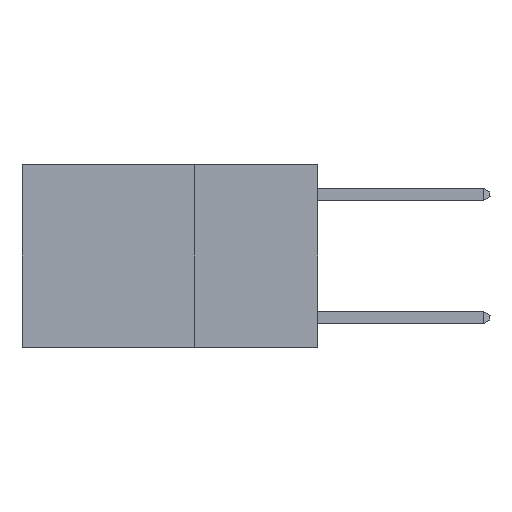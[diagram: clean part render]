
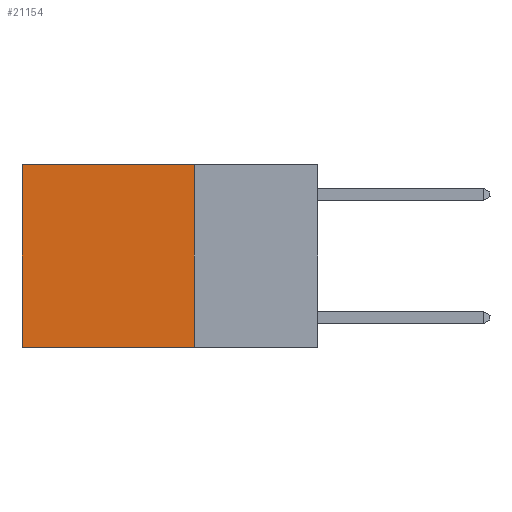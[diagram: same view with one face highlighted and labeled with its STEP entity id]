
A CAD part, left-side view. The second image highlights one B-rep face of the part: STEP entity #21154.
In plain terms, the highlighted planar face has unit normal (-1, 0, 0).
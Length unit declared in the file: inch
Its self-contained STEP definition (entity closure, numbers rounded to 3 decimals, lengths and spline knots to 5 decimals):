
#1165 = VECTOR ( 'NONE', #25791, 39.37008 ) ;
#1932 = VERTEX_POINT ( 'NONE', #30349 ) ;
#2267 = DIRECTION ( 'NONE',  ( 1., 0., 0. ) ) ;
#3977 = LINE ( 'NONE', #15741, #16238 ) ;
#4914 = LINE ( 'NONE', #23691, #30261 ) ;
#5158 = CARTESIAN_POINT ( 'NONE',  ( 0.2625, 0.6, -0.37 ) ) ;
#5174 = VERTEX_POINT ( 'NONE', #22373 ) ;
#7076 = ORIENTED_EDGE ( 'NONE', *, *, #25683, .F. ) ;
#7470 = ORIENTED_EDGE ( 'NONE', *, *, #29866, .T. ) ;
#8504 = VERTEX_POINT ( 'NONE', #5158 ) ;
#8608 = EDGE_CURVE ( 'NONE', #1932, #28725, #10724, .T. ) ;
#9175 = AXIS2_PLACEMENT_3D ( 'NONE', #31660, #2267, #19341 ) ;
#9919 = CARTESIAN_POINT ( 'NONE',  ( 0.2625, 0.6, 0. ) ) ;
#10724 = LINE ( 'NONE', #12882, #29503 ) ;
#12882 = CARTESIAN_POINT ( 'NONE',  ( 0.2625, 0.25, 0. ) ) ;
#14474 = PLANE ( 'NONE',  #9175 ) ;
#15741 = CARTESIAN_POINT ( 'NONE',  ( 0.2625, 0.25, -0.37 ) ) ;
#16238 = VECTOR ( 'NONE', #25462, 39.37008 ) ;
#17772 = DIRECTION ( 'NONE',  ( 0., 1., 0. ) ) ;
#18235 = ORIENTED_EDGE ( 'NONE', *, *, #29094, .F. ) ;
#19341 = DIRECTION ( 'NONE',  ( 0., 0., -1. ) ) ;
#21154 = ADVANCED_FACE ( 'NONE', ( #27954 ), #14474, .F. ) ;
#22373 = CARTESIAN_POINT ( 'NONE',  ( 0.2625, 0.25, -0.37 ) ) ;
#23691 = CARTESIAN_POINT ( 'NONE',  ( 0.2625, 0.6, 0. ) ) ;
#25462 = DIRECTION ( 'NONE',  ( 0., 1., 0. ) ) ;
#25683 = EDGE_CURVE ( 'NONE', #5174, #8504, #3977, .T. ) ;
#25791 = DIRECTION ( 'NONE',  ( 0., 0., -1. ) ) ;
#26390 = LINE ( 'NONE', #30804, #1165 ) ;
#27357 = EDGE_LOOP ( 'NONE', ( #7470, #7076, #18235, #29042 ) ) ;
#27954 = FACE_OUTER_BOUND ( 'NONE', #27357, .T. ) ;
#28725 = VERTEX_POINT ( 'NONE', #9919 ) ;
#29042 = ORIENTED_EDGE ( 'NONE', *, *, #8608, .T. ) ;
#29094 = EDGE_CURVE ( 'NONE', #1932, #5174, #26390, .T. ) ;
#29503 = VECTOR ( 'NONE', #17772, 39.37008 ) ;
#29866 = EDGE_CURVE ( 'NONE', #28725, #8504, #4914, .T. ) ;
#30261 = VECTOR ( 'NONE', #31208, 39.37008 ) ;
#30349 = CARTESIAN_POINT ( 'NONE',  ( 0.2625, 0.25, 0. ) ) ;
#30804 = CARTESIAN_POINT ( 'NONE',  ( 0.2625, 0.25, 0. ) ) ;
#31208 = DIRECTION ( 'NONE',  ( 0., 0., -1. ) ) ;
#31660 = CARTESIAN_POINT ( 'NONE',  ( 0.2625, 0.25, 0. ) ) ;
